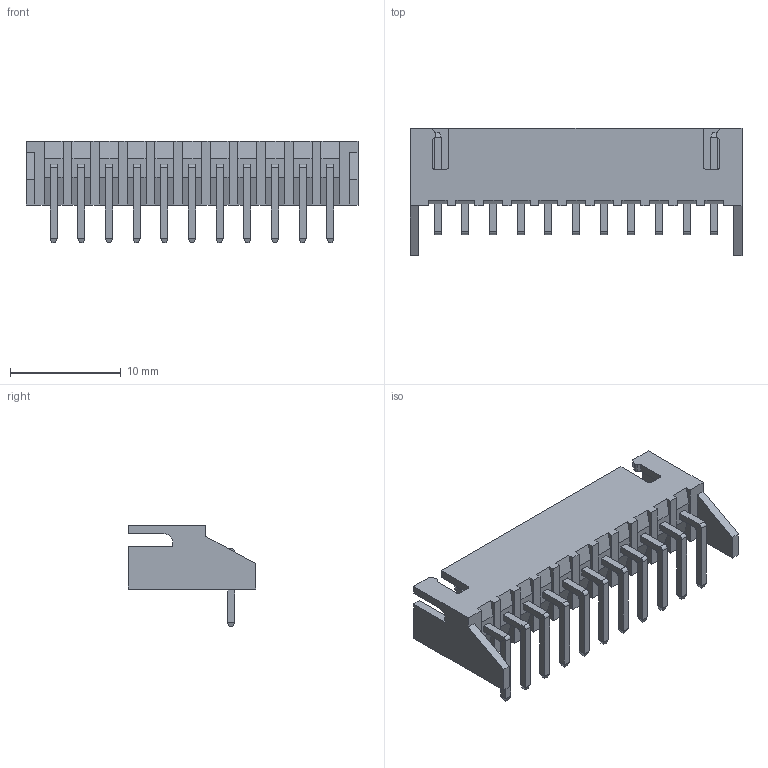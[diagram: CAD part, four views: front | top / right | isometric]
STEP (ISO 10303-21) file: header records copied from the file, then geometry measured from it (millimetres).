
FILE_DESCRIPTION (( 'STEP AP203' ), '1' );
FILE_NAME ('14K-511-416-AD1.STEP', '2024-02-22T15:44:50', ( '' ), ( '' ), 'SwSTEP 2.0', 'SolidWorks 2023', '' );
FILE_SCHEMA (( 'CONFIG_CONTROL_DESIGN' ));
Length unit declared in the file: millimetre
Products named in the file (3): 14K Series Pin with Stabilizer_16; 14K-511-416-AD1; 14K Series Pin Header Insulator with Stabilizer_511
Assembly tree (12 placements, depth 2):
  14K-511-416-AD1
    14K Series Pin Header Insulator with Stabilizer_511
    14K Series Pin with Stabilizer_16  x11
Bounding box: 30 x 11.5 x 9.15 mm (x, y, z)
Volume: 606.4 mm3; surface area: 1749.3 mm2
Topology: 12 solids, 12 shells, 398 faces, 1034 edges, 660 vertices
Faces by surface type: plane 367, cylinder 31
Entity records: 6409 total; most frequent: CARTESIAN_POINT 1047, ORIENTED_EDGE 1028, DIRECTION 926, EDGE_CURVE 514, VECTOR 488, LINE 488, VERTEX_POINT 340, AXIS2_PLACEMENT_3D 219
